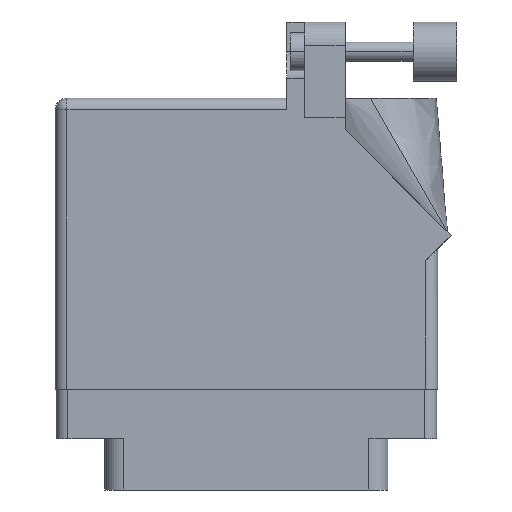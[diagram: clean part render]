
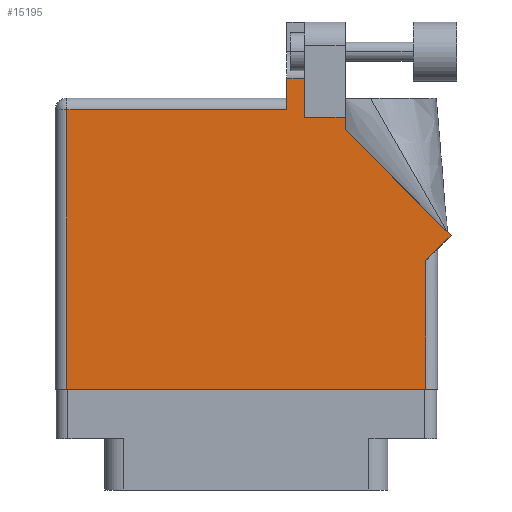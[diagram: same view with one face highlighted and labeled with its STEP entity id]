
A CAD part, front view. The second image highlights one B-rep face of the part: STEP entity #15195.
In plain terms, the highlighted face is planar.
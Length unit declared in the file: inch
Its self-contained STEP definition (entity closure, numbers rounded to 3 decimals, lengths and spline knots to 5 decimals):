
#625 = DIRECTION ( 'NONE',  ( 0.707, 0.707, 0. ) ) ;
#1077 = EDGE_CURVE ( 'NONE', #9712, #3615, #24185, .T. ) ;
#1909 = VERTEX_POINT ( 'NONE', #16340 ) ;
#2046 = DIRECTION ( 'NONE',  ( 0., 0., -1. ) ) ;
#2061 = CARTESIAN_POINT ( 'NONE',  ( 1.311, 1.43, 0. ) ) ;
#2065 = DIRECTION ( 'NONE',  ( 0., 1., 0. ) ) ;
#2302 = LINE ( 'NONE', #21674, #5294 ) ;
#2758 = VECTOR ( 'NONE', #19692, 39.37008 ) ;
#3010 = LINE ( 'NONE', #8243, #20413 ) ;
#3081 = CARTESIAN_POINT ( 'NONE',  ( 1.217, 1.468, 0. ) ) ;
#3119 = EDGE_CURVE ( 'NONE', #7326, #10652, #21019, .T. ) ;
#3453 = VECTOR ( 'NONE', #625, 39.37008 ) ;
#3615 = VERTEX_POINT ( 'NONE', #28161 ) ;
#3850 = ORIENTED_EDGE ( 'NONE', *, *, #34807, .T. ) ;
#4334 = CARTESIAN_POINT ( 'NONE',  ( 1.524, 1.36442, 0. ) ) ;
#4487 = AXIS2_PLACEMENT_3D ( 'NONE', #8548, #2046, #21933 ) ;
#5294 = VECTOR ( 'NONE', #29847, 39.37008 ) ;
#5404 = EDGE_CURVE ( 'NONE', #31290, #9384, #10197, .T. ) ;
#6403 = ORIENTED_EDGE ( 'NONE', *, *, #34006, .T. ) ;
#7326 = VERTEX_POINT ( 'NONE', #33651 ) ;
#7483 = DIRECTION ( 'NONE',  ( 1., 0., 0. ) ) ;
#8140 = ORIENTED_EDGE ( 'NONE', *, *, #17367, .T. ) ;
#8243 = CARTESIAN_POINT ( 'NONE',  ( 1.948, 0.737, 0. ) ) ;
#8548 = CARTESIAN_POINT ( 'NONE',  ( 0., 1.53, 0. ) ) ;
#9384 = VERTEX_POINT ( 'NONE', #33540 ) ;
#9712 = VERTEX_POINT ( 'NONE', #4334 ) ;
#9948 = LINE ( 'NONE', #22068, #2758 ) ;
#10197 = LINE ( 'NONE', #32859, #3453 ) ;
#10652 = VERTEX_POINT ( 'NONE', #16071 ) ;
#11257 = LINE ( 'NONE', #33153, #32657 ) ;
#12813 = EDGE_CURVE ( 'NONE', #1909, #15153, #9948, .T. ) ;
#13317 = CARTESIAN_POINT ( 'NONE',  ( 1.64177, 1.6315, 0. ) ) ;
#14978 = LINE ( 'NONE', #34589, #19651 ) ;
#15153 = VERTEX_POINT ( 'NONE', #27002 ) ;
#15195 = ADVANCED_FACE ( 'NONE', ( #19421 ), #15701, .F. ) ;
#15701 = PLANE ( 'NONE',  #4487 ) ;
#15976 = EDGE_CURVE ( 'NONE', #10652, #34146, #11257, .T. ) ;
#16071 = CARTESIAN_POINT ( 'NONE',  ( 1.217, 1.6315, 0. ) ) ;
#16340 = CARTESIAN_POINT ( 'NONE',  ( 0.062, 1.468, 0. ) ) ;
#16865 = EDGE_CURVE ( 'NONE', #3615, #31193, #30862, .T. ) ;
#17367 = EDGE_CURVE ( 'NONE', #34146, #1909, #2302, .T. ) ;
#19421 = FACE_OUTER_BOUND ( 'NONE', #32524, .T. ) ;
#19601 = CARTESIAN_POINT ( 'NONE',  ( 2.08071, 0.80771, 0. ) ) ;
#19651 = VECTOR ( 'NONE', #26819, 39.37008 ) ;
#19692 = DIRECTION ( 'NONE',  ( 0., -1., 0. ) ) ;
#19742 = VECTOR ( 'NONE', #29694, 39.37008 ) ;
#20413 = VECTOR ( 'NONE', #2065, 39.37008 ) ;
#20882 = CARTESIAN_POINT ( 'NONE',  ( 1.524, 1.36442, 0. ) ) ;
#20949 = ORIENTED_EDGE ( 'NONE', *, *, #16865, .T. ) ;
#21019 = LINE ( 'NONE', #13317, #19742 ) ;
#21107 = DIRECTION ( 'NONE',  ( 0., 1., 0. ) ) ;
#21469 = ORIENTED_EDGE ( 'NONE', *, *, #34600, .T. ) ;
#21674 = CARTESIAN_POINT ( 'NONE',  ( 0., 1.468, 0. ) ) ;
#21933 = DIRECTION ( 'NONE',  ( -1., 0., 0. ) ) ;
#22068 = CARTESIAN_POINT ( 'NONE',  ( 0.062, 0., 0. ) ) ;
#22110 = VECTOR ( 'NONE', #25007, 39.37008 ) ;
#22266 = VECTOR ( 'NONE', #25678, 39.37008 ) ;
#23058 = ORIENTED_EDGE ( 'NONE', *, *, #5404, .T. ) ;
#23407 = LINE ( 'NONE', #19601, #22110 ) ;
#23475 = VECTOR ( 'NONE', #7483, 39.37008 ) ;
#24185 = LINE ( 'NONE', #20882, #33165 ) ;
#24259 = CARTESIAN_POINT ( 'NONE',  ( 1.948, 0.675, 0. ) ) ;
#25007 = DIRECTION ( 'NONE',  ( -0.707, 0.707, 0. ) ) ;
#25678 = DIRECTION ( 'NONE',  ( -1., 0., 0. ) ) ;
#26553 = CARTESIAN_POINT ( 'NONE',  ( 0., 0., 0. ) ) ;
#26819 = DIRECTION ( 'NONE',  ( 0., 1., 0. ) ) ;
#26958 = ORIENTED_EDGE ( 'NONE', *, *, #1077, .T. ) ;
#26981 = ORIENTED_EDGE ( 'NONE', *, *, #33332, .T. ) ;
#27002 = CARTESIAN_POINT ( 'NONE',  ( 0.062, 0., 0. ) ) ;
#28161 = CARTESIAN_POINT ( 'NONE',  ( 1.524, 1.43, 0. ) ) ;
#29694 = DIRECTION ( 'NONE',  ( -1., 0., 0. ) ) ;
#29847 = DIRECTION ( 'NONE',  ( -1., 0., 0. ) ) ;
#30175 = CARTESIAN_POINT ( 'NONE',  ( 1.948, 0., 0. ) ) ;
#30660 = ORIENTED_EDGE ( 'NONE', *, *, #15976, .T. ) ;
#30862 = LINE ( 'NONE', #33309, #22266 ) ;
#31193 = VERTEX_POINT ( 'NONE', #2061 ) ;
#31260 = ORIENTED_EDGE ( 'NONE', *, *, #12813, .T. ) ;
#31290 = VERTEX_POINT ( 'NONE', #24259 ) ;
#31921 = VERTEX_POINT ( 'NONE', #30175 ) ;
#32524 = EDGE_LOOP ( 'NONE', ( #26981, #32999, #30660, #8140, #31260, #6403, #21469, #23058, #3850, #26958, #20949 ) ) ;
#32657 = VECTOR ( 'NONE', #33392, 39.37008 ) ;
#32859 = CARTESIAN_POINT ( 'NONE',  ( 2.01, 0.737, 0. ) ) ;
#32873 = LINE ( 'NONE', #26553, #23475 ) ;
#32999 = ORIENTED_EDGE ( 'NONE', *, *, #3119, .T. ) ;
#33153 = CARTESIAN_POINT ( 'NONE',  ( 1.217, 1.53, 0. ) ) ;
#33165 = VECTOR ( 'NONE', #21107, 39.37008 ) ;
#33309 = CARTESIAN_POINT ( 'NONE',  ( 1.524, 1.43, 0. ) ) ;
#33332 = EDGE_CURVE ( 'NONE', #31193, #7326, #14978, .T. ) ;
#33392 = DIRECTION ( 'NONE',  ( 0., -1., 0. ) ) ;
#33540 = CARTESIAN_POINT ( 'NONE',  ( 2.08071, 0.80771, 0. ) ) ;
#33651 = CARTESIAN_POINT ( 'NONE',  ( 1.311, 1.6315, 0. ) ) ;
#34006 = EDGE_CURVE ( 'NONE', #15153, #31921, #32873, .T. ) ;
#34146 = VERTEX_POINT ( 'NONE', #3081 ) ;
#34589 = CARTESIAN_POINT ( 'NONE',  ( 1.311, 1.43, 0. ) ) ;
#34600 = EDGE_CURVE ( 'NONE', #31921, #31290, #3010, .T. ) ;
#34807 = EDGE_CURVE ( 'NONE', #9384, #9712, #23407, .T. ) ;
